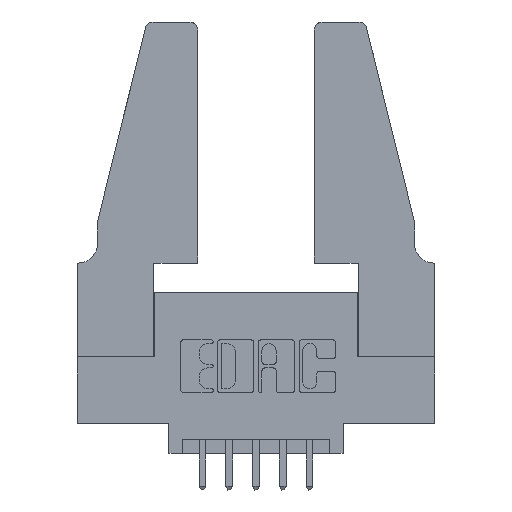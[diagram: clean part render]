
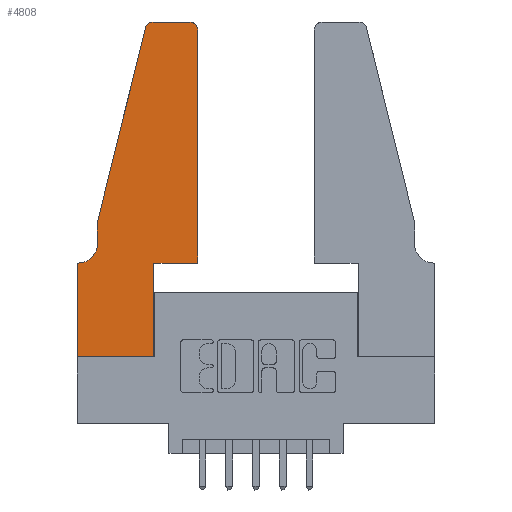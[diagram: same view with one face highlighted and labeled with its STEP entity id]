
A CAD part, top view. The second image highlights one B-rep face of the part: STEP entity #4808.
In plain terms, the highlighted planar face has unit normal (0, 0, 1).
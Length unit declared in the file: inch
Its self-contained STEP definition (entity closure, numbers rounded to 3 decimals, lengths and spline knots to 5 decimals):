
#167 = CARTESIAN_POINT ( 'NONE',  ( 0., 0.35, 0.37 ) ) ;
#272 = ORIENTED_EDGE ( 'NONE', *, *, #1762, .T. ) ;
#325 = EDGE_CURVE ( 'NONE', #596, #6010, #9704, .T. ) ;
#596 = VERTEX_POINT ( 'NONE', #4986 ) ;
#810 = VERTEX_POINT ( 'NONE', #4453 ) ;
#879 = AXIS2_PLACEMENT_3D ( 'NONE', #8355, #8387, #7899 ) ;
#950 = CARTESIAN_POINT ( 'NONE',  ( 0.4205, 1.25, 0.37 ) ) ;
#1015 = EDGE_CURVE ( 'NONE', #1702, #1186, #3295, .T. ) ;
#1038 = EDGE_CURVE ( 'NONE', #2668, #1702, #5366, .T. ) ;
#1136 = DIRECTION ( 'NONE',  ( 0., 0., 1. ) ) ;
#1165 = CARTESIAN_POINT ( 'NONE',  ( 0.0055, 0.35, 0.37 ) ) ;
#1176 = CARTESIAN_POINT ( 'NONE',  ( 0.0755, 0.42, 0.37 ) ) ;
#1186 = VERTEX_POINT ( 'NONE', #4791 ) ;
#1201 = EDGE_LOOP ( 'NONE', ( #4877, #2821, #5432, #9875, #7951, #6244, #1878, #4205, #10965, #2413, #9251, #272 ) ) ;
#1341 = CARTESIAN_POINT ( 'NONE',  ( 0.284, 1.25, 0.37 ) ) ;
#1553 = CARTESIAN_POINT ( 'NONE',  ( 0.2865, 0.35, 0.37 ) ) ;
#1643 = VECTOR ( 'NONE', #7466, 39.37008 ) ;
#1702 = VERTEX_POINT ( 'NONE', #6150 ) ;
#1762 = EDGE_CURVE ( 'NONE', #6010, #9076, #5648, .T. ) ;
#1793 = VECTOR ( 'NONE', #8311, 39.37008 ) ;
#1878 = ORIENTED_EDGE ( 'NONE', *, *, #1015, .T. ) ;
#2007 = EDGE_CURVE ( 'NONE', #2088, #3218, #5509, .T. ) ;
#2088 = VERTEX_POINT ( 'NONE', #1341 ) ;
#2335 = CARTESIAN_POINT ( 'NONE',  ( 0.0755, 0.5, 0.37 ) ) ;
#2365 = CARTESIAN_POINT ( 'NONE',  ( 0.0755, 0.35, 0.37 ) ) ;
#2413 = ORIENTED_EDGE ( 'NONE', *, *, #5874, .T. ) ;
#2453 = VECTOR ( 'NONE', #7238, 39.37008 ) ;
#2574 = DIRECTION ( 'NONE',  ( 1., 0., 0. ) ) ;
#2668 = VERTEX_POINT ( 'NONE', #1165 ) ;
#2821 = ORIENTED_EDGE ( 'NONE', *, *, #2007, .T. ) ;
#2912 = VECTOR ( 'NONE', #4971, 39.37008 ) ;
#3026 = VECTOR ( 'NONE', #5426, 39.37008 ) ;
#3169 = CIRCLE ( 'NONE', #7864, 0.07 ) ;
#3184 = EDGE_CURVE ( 'NONE', #1186, #810, #9527, .T. ) ;
#3218 = VERTEX_POINT ( 'NONE', #7139 ) ;
#3272 = EDGE_CURVE ( 'NONE', #810, #5762, #8506, .T. ) ;
#3295 = LINE ( 'NONE', #5466, #5901 ) ;
#3354 = LINE ( 'NONE', #10265, #7689 ) ;
#4060 = CARTESIAN_POINT ( 'NONE',  ( 0.4505, 0.35, 0.37 ) ) ;
#4205 = ORIENTED_EDGE ( 'NONE', *, *, #3184, .T. ) ;
#4453 = CARTESIAN_POINT ( 'NONE',  ( 0.2865, 0., 0.37 ) ) ;
#4534 = CARTESIAN_POINT ( 'NONE',  ( 0.0055, 0.42, 0.37 ) ) ;
#4761 = FACE_OUTER_BOUND ( 'NONE', #1201, .T. ) ;
#4791 = CARTESIAN_POINT ( 'NONE',  ( 0., 0., 0.37 ) ) ;
#4795 = EDGE_CURVE ( 'NONE', #6819, #10235, #9269, .T. ) ;
#4808 = ADVANCED_FACE ( 'NONE', ( #4761 ), #5525, .T. ) ;
#4877 = ORIENTED_EDGE ( 'NONE', *, *, #10244, .T. ) ;
#4890 = CARTESIAN_POINT ( 'NONE',  ( 0.0755, 0.5, 0.37 ) ) ;
#4971 = DIRECTION ( 'NONE',  ( 0., 1., 0. ) ) ;
#4986 = CARTESIAN_POINT ( 'NONE',  ( 0.4505, 0.35, 0.37 ) ) ;
#5320 = VECTOR ( 'NONE', #7200, 39.37008 ) ;
#5366 = LINE ( 'NONE', #2365, #3026 ) ;
#5411 = DIRECTION ( 'NONE',  ( -1., 0., 0. ) ) ;
#5414 = AXIS2_PLACEMENT_3D ( 'NONE', #167, #1136, #7239 ) ;
#5426 = DIRECTION ( 'NONE',  ( -1., 0., 0. ) ) ;
#5432 = ORIENTED_EDGE ( 'NONE', *, *, #10409, .T. ) ;
#5466 = CARTESIAN_POINT ( 'NONE',  ( 0., 0., 0.37 ) ) ;
#5494 = DIRECTION ( 'NONE',  ( 0., -1., 0. ) ) ;
#5509 = CIRCLE ( 'NONE', #879, 0.03 ) ;
#5525 = PLANE ( 'NONE',  #5414 ) ;
#5648 = CIRCLE ( 'NONE', #11097, 0.03 ) ;
#5762 = VERTEX_POINT ( 'NONE', #1553 ) ;
#5826 = DIRECTION ( 'NONE',  ( 1., 0., 0. ) ) ;
#5838 = DIRECTION ( 'NONE',  ( 0., 0., 1. ) ) ;
#5848 = CARTESIAN_POINT ( 'NONE',  ( 0.4205, 1.22, 0.37 ) ) ;
#5874 = EDGE_CURVE ( 'NONE', #5762, #596, #3354, .T. ) ;
#5901 = VECTOR ( 'NONE', #5494, 39.37008 ) ;
#6010 = VERTEX_POINT ( 'NONE', #10602 ) ;
#6024 = LINE ( 'NONE', #8937, #6414 ) ;
#6150 = CARTESIAN_POINT ( 'NONE',  ( 0., 0.35, 0.37 ) ) ;
#6244 = ORIENTED_EDGE ( 'NONE', *, *, #1038, .T. ) ;
#6414 = VECTOR ( 'NONE', #9748, 39.37008 ) ;
#6428 = LINE ( 'NONE', #4890, #1793 ) ;
#6819 = VERTEX_POINT ( 'NONE', #2335 ) ;
#7139 = CARTESIAN_POINT ( 'NONE',  ( 0.25487, 1.22718, 0.37 ) ) ;
#7200 = DIRECTION ( 'NONE',  ( 0., -1., 0. ) ) ;
#7209 = CARTESIAN_POINT ( 'NONE',  ( 0., 0., 0.37 ) ) ;
#7238 = DIRECTION ( 'NONE',  ( 1., 0., 0. ) ) ;
#7239 = DIRECTION ( 'NONE',  ( 1., 0., 0. ) ) ;
#7280 = CARTESIAN_POINT ( 'NONE',  ( 0.2865, 0.35, 0.37 ) ) ;
#7466 = DIRECTION ( 'NONE',  ( 0., 1., 0. ) ) ;
#7689 = VECTOR ( 'NONE', #2574, 39.37008 ) ;
#7864 = AXIS2_PLACEMENT_3D ( 'NONE', #4534, #10444, #5411 ) ;
#7899 = DIRECTION ( 'NONE',  ( 1., 0., 0. ) ) ;
#7906 = EDGE_CURVE ( 'NONE', #10235, #2668, #3169, .T. ) ;
#7951 = ORIENTED_EDGE ( 'NONE', *, *, #7906, .T. ) ;
#8035 = CARTESIAN_POINT ( 'NONE',  ( 0.0755, 0.5, 0.37 ) ) ;
#8311 = DIRECTION ( 'NONE',  ( -0.239, -0.971, 0. ) ) ;
#8355 = CARTESIAN_POINT ( 'NONE',  ( 0.284, 1.22, 0.37 ) ) ;
#8387 = DIRECTION ( 'NONE',  ( 0., 0., 1. ) ) ;
#8506 = LINE ( 'NONE', #7280, #1643 ) ;
#8937 = CARTESIAN_POINT ( 'NONE',  ( 0.2605, 1.25, 0.37 ) ) ;
#9076 = VERTEX_POINT ( 'NONE', #950 ) ;
#9251 = ORIENTED_EDGE ( 'NONE', *, *, #325, .T. ) ;
#9269 = LINE ( 'NONE', #8035, #5320 ) ;
#9527 = LINE ( 'NONE', #7209, #2453 ) ;
#9704 = LINE ( 'NONE', #4060, #2912 ) ;
#9748 = DIRECTION ( 'NONE',  ( -1., 0., 0. ) ) ;
#9875 = ORIENTED_EDGE ( 'NONE', *, *, #4795, .T. ) ;
#10235 = VERTEX_POINT ( 'NONE', #1176 ) ;
#10244 = EDGE_CURVE ( 'NONE', #9076, #2088, #6024, .T. ) ;
#10265 = CARTESIAN_POINT ( 'NONE',  ( 0.4505, 0.35, 0.37 ) ) ;
#10409 = EDGE_CURVE ( 'NONE', #3218, #6819, #6428, .T. ) ;
#10444 = DIRECTION ( 'NONE',  ( 0., 0., -1. ) ) ;
#10602 = CARTESIAN_POINT ( 'NONE',  ( 0.4505, 1.22, 0.37 ) ) ;
#10965 = ORIENTED_EDGE ( 'NONE', *, *, #3272, .T. ) ;
#11097 = AXIS2_PLACEMENT_3D ( 'NONE', #5848, #5838, #5826 ) ;
